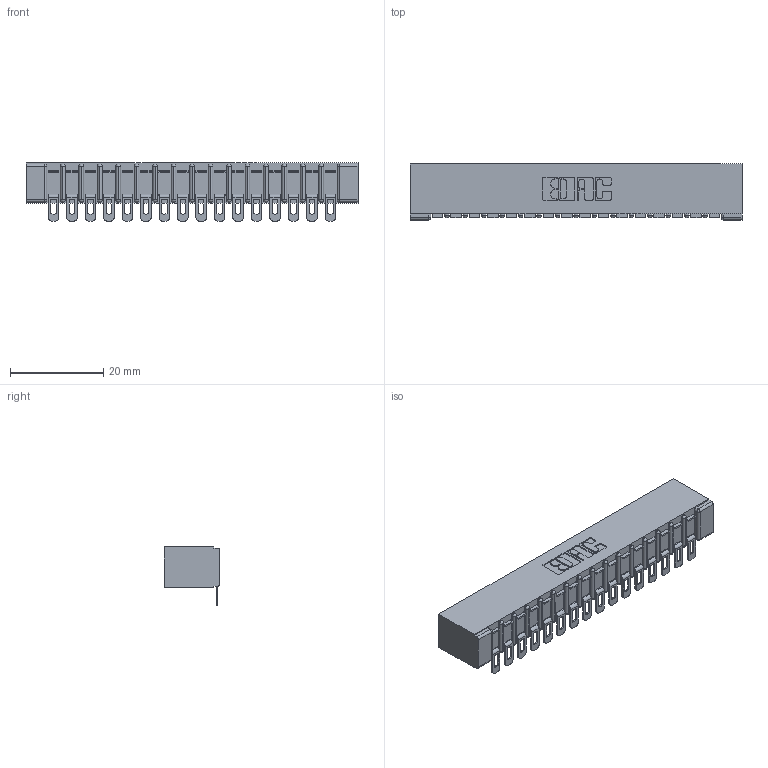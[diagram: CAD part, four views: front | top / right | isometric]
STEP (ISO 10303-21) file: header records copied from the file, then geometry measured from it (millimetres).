
FILE_DESCRIPTION (( 'STEP AP203' ), '1' );
FILE_NAME ('357-016-554-101.STEP', '2019-09-16T20:47:57', ( '' ), ( '' ), 'SwSTEP 2.0', 'SolidWorks 2016', '' );
FILE_SCHEMA (( 'CONFIG_CONTROL_DESIGN' ));
Length unit declared in the file: inch
Products named in the file (3): 307 Part_No Mounting Lugs; 307-290-002_554; 357-016-554-101
Assembly tree (17 placements, depth 2):
  357-016-554-101
    307 Part_No Mounting Lugs
    307-290-002_554  x16
Bounding box: 71.27 x 12.01 x 12.52 mm (x, y, z)
Volume: 4950.2 mm3; surface area: 9243 mm2
Topology: 17 solids, 17 shells, 1423 faces, 4347 edges, 2850 vertices
Faces by surface type: plane 802, cylinder 587, sphere 34
Entity records: 17609 total; most frequent: CARTESIAN_POINT 2966, ORIENTED_EDGE 2956, DIRECTION 2898, EDGE_CURVE 1478, LINE 1114, VECTOR 1114, VERTEX_POINT 960, AXIS2_PLACEMENT_3D 892
